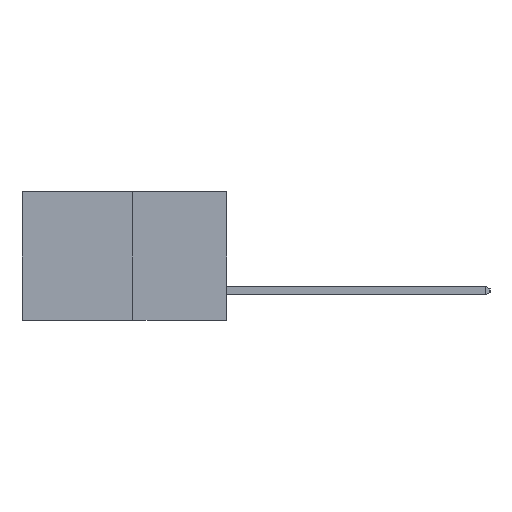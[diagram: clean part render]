
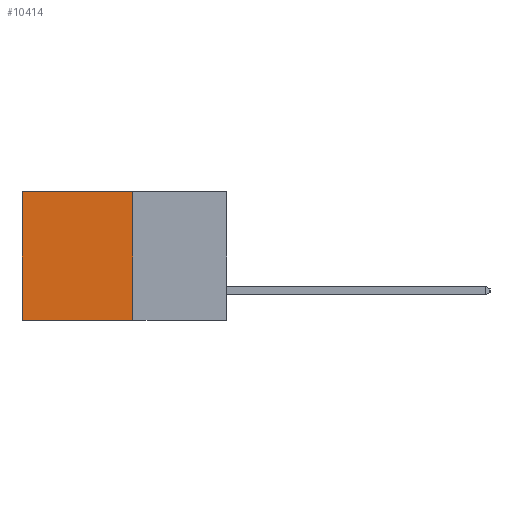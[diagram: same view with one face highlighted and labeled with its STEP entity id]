
A CAD part, left-side view. The second image highlights one B-rep face of the part: STEP entity #10414.
In plain terms, the highlighted planar face has unit normal (-1, 0, 0).
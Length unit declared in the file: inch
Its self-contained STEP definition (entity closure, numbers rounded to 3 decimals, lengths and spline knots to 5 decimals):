
#343 = ORIENTED_EDGE ( 'NONE', *, *, #991, .T. ) ;
#619 = VERTEX_POINT ( 'NONE', #8599 ) ;
#813 = CARTESIAN_POINT ( 'NONE',  ( 0.277, 0.27, 0. ) ) ;
#991 = EDGE_CURVE ( 'NONE', #8523, #619, #5832, .T. ) ;
#1251 = VECTOR ( 'NONE', #9466, 39.37008 ) ;
#2076 = CARTESIAN_POINT ( 'NONE',  ( 0.277, 0.27, -0.37 ) ) ;
#2477 = ORIENTED_EDGE ( 'NONE', *, *, #8221, .F. ) ;
#2727 = VERTEX_POINT ( 'NONE', #6032 ) ;
#3024 = VECTOR ( 'NONE', #9983, 39.37008 ) ;
#3068 = LINE ( 'NONE', #8496, #5127 ) ;
#3426 = VECTOR ( 'NONE', #9095, 39.37008 ) ;
#3764 = DIRECTION ( 'NONE',  ( 1., 0., 0. ) ) ;
#5127 = VECTOR ( 'NONE', #7577, 39.37008 ) ;
#5427 = CARTESIAN_POINT ( 'NONE',  ( 0.277, 0.27, -0.37 ) ) ;
#5621 = EDGE_CURVE ( 'NONE', #619, #8181, #7612, .T. ) ;
#5791 = EDGE_CURVE ( 'NONE', #8523, #2727, #7732, .T. ) ;
#5832 = LINE ( 'NONE', #7381, #1251 ) ;
#6032 = CARTESIAN_POINT ( 'NONE',  ( 0.277, 0.27, -0.37 ) ) ;
#6328 = PLANE ( 'NONE',  #10602 ) ;
#6578 = CARTESIAN_POINT ( 'NONE',  ( 0.277, 0.59, -0.37 ) ) ;
#6918 = EDGE_LOOP ( 'NONE', ( #9039, #2477, #7032, #343 ) ) ;
#7032 = ORIENTED_EDGE ( 'NONE', *, *, #5791, .F. ) ;
#7381 = CARTESIAN_POINT ( 'NONE',  ( 0.277, 0.27, 0. ) ) ;
#7577 = DIRECTION ( 'NONE',  ( 0., 1., 0. ) ) ;
#7612 = LINE ( 'NONE', #10017, #3024 ) ;
#7732 = LINE ( 'NONE', #5427, #3426 ) ;
#8181 = VERTEX_POINT ( 'NONE', #6578 ) ;
#8221 = EDGE_CURVE ( 'NONE', #2727, #8181, #3068, .T. ) ;
#8496 = CARTESIAN_POINT ( 'NONE',  ( 0.277, 0.27, -0.37 ) ) ;
#8523 = VERTEX_POINT ( 'NONE', #813 ) ;
#8599 = CARTESIAN_POINT ( 'NONE',  ( 0.277, 0.59, 0. ) ) ;
#9039 = ORIENTED_EDGE ( 'NONE', *, *, #5621, .T. ) ;
#9095 = DIRECTION ( 'NONE',  ( 0., 0., -1. ) ) ;
#9466 = DIRECTION ( 'NONE',  ( 0., 1., 0. ) ) ;
#9679 = FACE_OUTER_BOUND ( 'NONE', #6918, .T. ) ;
#9695 = DIRECTION ( 'NONE',  ( 0., 0., -1. ) ) ;
#9983 = DIRECTION ( 'NONE',  ( 0., 0., -1. ) ) ;
#10017 = CARTESIAN_POINT ( 'NONE',  ( 0.277, 0.59, -0.37 ) ) ;
#10414 = ADVANCED_FACE ( 'NONE', ( #9679 ), #6328, .F. ) ;
#10602 = AXIS2_PLACEMENT_3D ( 'NONE', #2076, #3764, #9695 ) ;
